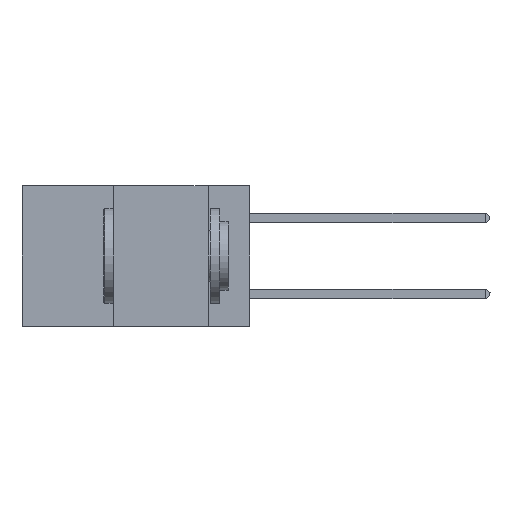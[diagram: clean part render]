
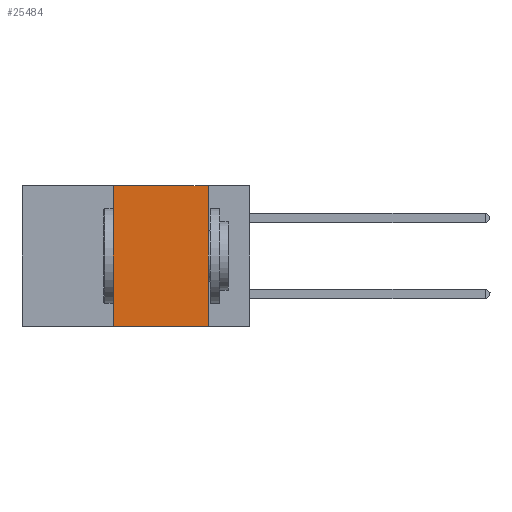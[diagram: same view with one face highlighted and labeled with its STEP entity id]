
A CAD part, left-side view. The second image highlights one B-rep face of the part: STEP entity #25484.
In plain terms, the highlighted planar face has unit normal (-1, 0, 0).
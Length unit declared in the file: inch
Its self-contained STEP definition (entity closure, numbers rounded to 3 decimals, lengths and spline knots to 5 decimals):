
#89 = LINE ( 'NONE', #41608, #35870 ) ;
#2177 = CARTESIAN_POINT ( 'NONE',  ( 0., 0.6, 0. ) ) ;
#2519 = FACE_OUTER_BOUND ( 'NONE', #8829, .T. ) ;
#5499 = CARTESIAN_POINT ( 'NONE',  ( 0., 0.11, -0.37 ) ) ;
#5721 = EDGE_CURVE ( 'NONE', #8906, #37385, #38697, .T. ) ;
#5781 = EDGE_CURVE ( 'NONE', #37385, #43220, #43638, .T. ) ;
#6183 = DIRECTION ( 'NONE',  ( 0., 0., -1. ) ) ;
#6917 = DIRECTION ( 'NONE',  ( 1., 0., 0. ) ) ;
#7827 = AXIS2_PLACEMENT_3D ( 'NONE', #31582, #6917, #31738 ) ;
#8829 = EDGE_LOOP ( 'NONE', ( #28445, #22385, #26798, #37333 ) ) ;
#8906 = VERTEX_POINT ( 'NONE', #41953 ) ;
#11417 = EDGE_CURVE ( 'NONE', #43220, #33776, #89, .T. ) ;
#16309 = LINE ( 'NONE', #17845, #36248 ) ;
#16647 = DIRECTION ( 'NONE',  ( 0., -1., 0. ) ) ;
#17845 = CARTESIAN_POINT ( 'NONE',  ( 0., 0.6, -0.37 ) ) ;
#21101 = PLANE ( 'NONE',  #7827 ) ;
#21808 = EDGE_CURVE ( 'NONE', #8906, #33776, #16309, .T. ) ;
#22385 = ORIENTED_EDGE ( 'NONE', *, *, #5781, .F. ) ;
#22849 = CARTESIAN_POINT ( 'NONE',  ( 0., 0.36, 0. ) ) ;
#24826 = VECTOR ( 'NONE', #16647, 39.37008 ) ;
#25484 = ADVANCED_FACE ( 'NONE', ( #2519 ), #21101, .F. ) ;
#26798 = ORIENTED_EDGE ( 'NONE', *, *, #5721, .F. ) ;
#28445 = ORIENTED_EDGE ( 'NONE', *, *, #11417, .F. ) ;
#30391 = CARTESIAN_POINT ( 'NONE',  ( 0., 0.36, 0. ) ) ;
#31582 = CARTESIAN_POINT ( 'NONE',  ( 0., 0.6, 0. ) ) ;
#31738 = DIRECTION ( 'NONE',  ( 0., 0., -1. ) ) ;
#33776 = VERTEX_POINT ( 'NONE', #5499 ) ;
#33956 = DIRECTION ( 'NONE',  ( 0., 0., 1. ) ) ;
#35523 = CARTESIAN_POINT ( 'NONE',  ( 0., 0.11, 0. ) ) ;
#35870 = VECTOR ( 'NONE', #6183, 39.37008 ) ;
#36248 = VECTOR ( 'NONE', #42574, 39.37008 ) ;
#37333 = ORIENTED_EDGE ( 'NONE', *, *, #21808, .T. ) ;
#37385 = VERTEX_POINT ( 'NONE', #22849 ) ;
#37570 = VECTOR ( 'NONE', #33956, 39.37008 ) ;
#38697 = LINE ( 'NONE', #30391, #37570 ) ;
#41608 = CARTESIAN_POINT ( 'NONE',  ( 0., 0.11, 0. ) ) ;
#41953 = CARTESIAN_POINT ( 'NONE',  ( 0., 0.36, -0.37 ) ) ;
#42574 = DIRECTION ( 'NONE',  ( 0., -1., 0. ) ) ;
#43220 = VERTEX_POINT ( 'NONE', #35523 ) ;
#43638 = LINE ( 'NONE', #2177, #24826 ) ;
